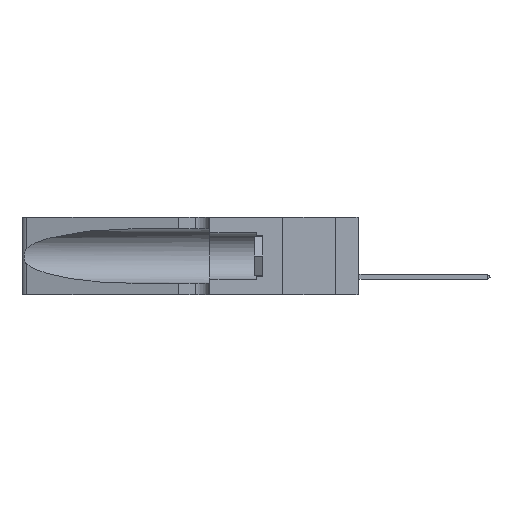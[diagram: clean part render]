
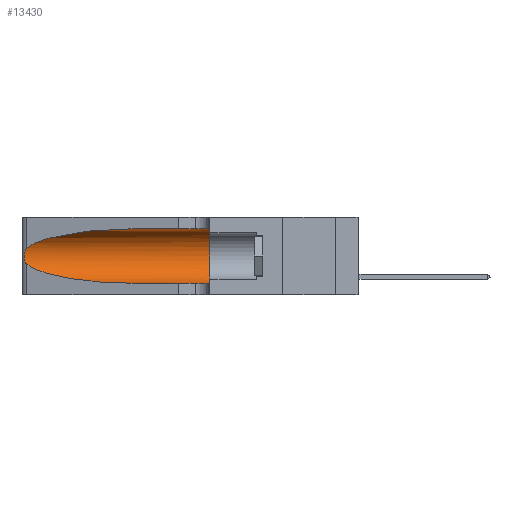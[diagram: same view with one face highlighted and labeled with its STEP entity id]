
A CAD part, left-side view. The second image highlights one B-rep face of the part: STEP entity #13430.
In plain terms, the highlighted cylindrical face has radius 3.308 mm (diameter 6.617 mm), a partial arc.
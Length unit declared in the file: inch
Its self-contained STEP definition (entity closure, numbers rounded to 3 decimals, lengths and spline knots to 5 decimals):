
#229 = CARTESIAN_POINT ( 'NONE',  ( 0.26017, 1.23833, 0.17102 ) ) ;
#629 = EDGE_CURVE ( 'NONE', #29864, #7412, #12571, .T. ) ;
#1246 = CARTESIAN_POINT ( 'NONE',  ( 0.25555, 1.22993, 0.14849 ) ) ;
#1469 = FACE_OUTER_BOUND ( 'NONE', #26520, .T. ) ;
#1801 = CARTESIAN_POINT ( 'NONE',  ( 0.1305, 0.72297, 0.05475 ) ) ;
#1826 = DIRECTION ( 'NONE',  ( 0., 0., -1. ) ) ;
#1872 = CARTESIAN_POINT ( 'NONE',  ( 0.25639, 1.23184, 0.21858 ) ) ;
#2039 = DIRECTION ( 'NONE',  ( 0., -1., 0. ) ) ;
#2766 = ORIENTED_EDGE ( 'NONE', *, *, #15524, .T. ) ;
#3517 = CARTESIAN_POINT ( 'NONE',  ( 0.25487, 1.22718, 0.14631 ) ) ;
#4753 = CARTESIAN_POINT ( 'NONE',  ( 0.26075, 1.23896, 0.19203 ) ) ;
#5401 = DIRECTION ( 'NONE',  ( 0., 1., 0. ) ) ;
#5763 = EDGE_CURVE ( 'NONE', #7412, #25248, #6986, .T. ) ;
#6132 = ORIENTED_EDGE ( 'NONE', *, *, #23559, .T. ) ;
#6464 = CARTESIAN_POINT ( 'NONE',  ( 0.25487, 1.22718, 0.22369 ) ) ;
#6986 = CIRCLE ( 'NONE', #9487, 0.13025 ) ;
#7412 = VERTEX_POINT ( 'NONE', #16437 ) ;
#8755 = CARTESIAN_POINT ( 'NONE',  ( 0.2373, 1.15595, 0.08982 ) ) ;
#9094 = ORIENTED_EDGE ( 'NONE', *, *, #629, .F. ) ;
#9487 = AXIS2_PLACEMENT_3D ( 'NONE', #20030, #5401, #25177 ) ;
#9727 = DIRECTION ( 'NONE',  ( 0., -1., 0. ) ) ;
#10022 =( BOUNDED_CURVE ( )  B_SPLINE_CURVE ( 3, ( #13956, #8755, #23247, #1801 ),
 .UNSPECIFIED., .F., .T. ) 
 B_SPLINE_CURVE_WITH_KNOTS ( ( 4, 4 ),
 ( 3.44316, 4.71239 ),
 .UNSPECIFIED. ) 
 CURVE ( )  GEOMETRIC_REPRESENTATION_ITEM ( )  RATIONAL_B_SPLINE_CURVE ( ( 1., 0.87, 0.87, 1. ) ) 
 REPRESENTATION_ITEM ( '' )  );
#10595 = DIRECTION ( 'NONE',  ( 0., -1., 0. ) ) ;
#10923 = EDGE_CURVE ( 'NONE', #16857, #25248, #27092, .T. ) ;
#11003 = CARTESIAN_POINT ( 'NONE',  ( 0.25639, 1.23186, 0.15144 ) ) ;
#11546 = CARTESIAN_POINT ( 'NONE',  ( 0.18966, 0.96281, 0.31525 ) ) ;
#12001 = CARTESIAN_POINT ( 'NONE',  ( 0.25555, 1.22994, 0.2215 ) ) ;
#12234 = CARTESIAN_POINT ( 'NONE',  ( 0.1305, 0.35, 0.05475 ) ) ;
#12571 = LINE ( 'NONE', #26975, #15242 ) ;
#12709 = VERTEX_POINT ( 'NONE', #3517 ) ;
#13430 = ADVANCED_FACE ( 'NONE', ( #1469 ), #29130, .F. ) ;
#13672 = CARTESIAN_POINT ( 'NONE',  ( 0.2373, 1.15595, 0.28018 ) ) ;
#13687 = CARTESIAN_POINT ( 'NONE',  ( 0.1305, 0.72297, 0.05475 ) ) ;
#13956 = CARTESIAN_POINT ( 'NONE',  ( 0.25487, 1.22718, 0.14631 ) ) ;
#14637 = CARTESIAN_POINT ( 'NONE',  ( 0.25854, 1.2359, 0.20912 ) ) ;
#14727 = VERTEX_POINT ( 'NONE', #21059 ) ;
#14836 = CARTESIAN_POINT ( 'NONE',  ( 0.26075, 1.23896, 0.178 ) ) ;
#15242 = VECTOR ( 'NONE', #9727, 39.37008 ) ;
#15524 = EDGE_CURVE ( 'NONE', #29864, #14727, #17203, .T. ) ;
#16437 = CARTESIAN_POINT ( 'NONE',  ( 0.1305, 0.35, 0.31525 ) ) ;
#16857 = VERTEX_POINT ( 'NONE', #13687 ) ;
#17036 = ORIENTED_EDGE ( 'NONE', *, *, #10923, .T. ) ;
#17203 =( BOUNDED_CURVE ( )  B_SPLINE_CURVE ( 3, ( #18658, #11546, #13672, #6464 ),
 .UNSPECIFIED., .F., .F. ) 
 B_SPLINE_CURVE_WITH_KNOTS ( ( 4, 4 ),
 ( 1.5708, 2.84003 ),
 .UNSPECIFIED. ) 
 CURVE ( )  GEOMETRIC_REPRESENTATION_ITEM ( )  RATIONAL_B_SPLINE_CURVE ( ( 1., 0.87, 0.87, 1. ) ) 
 REPRESENTATION_ITEM ( '' )  );
#17890 = ORIENTED_EDGE ( 'NONE', *, *, #5763, .F. ) ;
#17903 = CARTESIAN_POINT ( 'NONE',  ( 0.1305, 1.61858, 0.05475 ) ) ;
#18658 = CARTESIAN_POINT ( 'NONE',  ( 0.1305, 0.72297, 0.31525 ) ) ;
#18794 = CARTESIAN_POINT ( 'NONE',  ( 0.25487, 1.22718, 0.22369 ) ) ;
#20030 = CARTESIAN_POINT ( 'NONE',  ( 0.1305, 0.35, 0.185 ) ) ;
#21043 = VECTOR ( 'NONE', #10595, 39.37008 ) ;
#21059 = CARTESIAN_POINT ( 'NONE',  ( 0.25487, 1.22718, 0.22369 ) ) ;
#21800 = CARTESIAN_POINT ( 'NONE',  ( 0.25856, 1.23593, 0.16098 ) ) ;
#21998 = CARTESIAN_POINT ( 'NONE',  ( 0.26018, 1.23835, 0.19895 ) ) ;
#22240 = B_SPLINE_CURVE_WITH_KNOTS ( 'NONE', 3,
 ( #18794, #12001, #1872, #23705, #14637, #21998, #4753, #14836, #229, #21800, #29748, #11003, #1246, #27223 ),
 .UNSPECIFIED., .F., .F.,
 ( 4, 2, 2, 2, 2, 2, 4 ),
 ( 0., 0.00027, 0.00053, 0.00107, 0.0016, 0.00187, 0.00214 ),
 .UNSPECIFIED. ) ;
#23247 = CARTESIAN_POINT ( 'NONE',  ( 0.18966, 0.96281, 0.05475 ) ) ;
#23559 = EDGE_CURVE ( 'NONE', #14727, #12709, #22240, .T. ) ;
#23560 = CARTESIAN_POINT ( 'NONE',  ( 0.1305, 1.61858, 0.185 ) ) ;
#23705 = CARTESIAN_POINT ( 'NONE',  ( 0.25787, 1.23484, 0.2124 ) ) ;
#25177 = DIRECTION ( 'NONE',  ( 0., 0., 1. ) ) ;
#25248 = VERTEX_POINT ( 'NONE', #12234 ) ;
#25894 = EDGE_CURVE ( 'NONE', #12709, #16857, #10022, .T. ) ;
#26520 = EDGE_LOOP ( 'NONE', ( #2766, #6132, #31072, #17036, #17890, #9094 ) ) ;
#26975 = CARTESIAN_POINT ( 'NONE',  ( 0.1305, 1.61858, 0.31525 ) ) ;
#27092 = LINE ( 'NONE', #17903, #21043 ) ;
#27198 = AXIS2_PLACEMENT_3D ( 'NONE', #23560, #2039, #1826 ) ;
#27223 = CARTESIAN_POINT ( 'NONE',  ( 0.25487, 1.22718, 0.14631 ) ) ;
#29130 = CYLINDRICAL_SURFACE ( 'NONE', #27198, 0.13025 ) ;
#29748 = CARTESIAN_POINT ( 'NONE',  ( 0.25789, 1.23486, 0.15765 ) ) ;
#29864 = VERTEX_POINT ( 'NONE', #29997 ) ;
#29997 = CARTESIAN_POINT ( 'NONE',  ( 0.1305, 0.72297, 0.31525 ) ) ;
#31072 = ORIENTED_EDGE ( 'NONE', *, *, #25894, .T. ) ;
